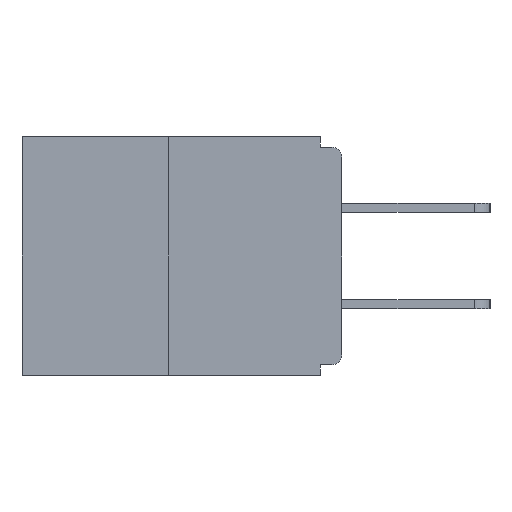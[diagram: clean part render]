
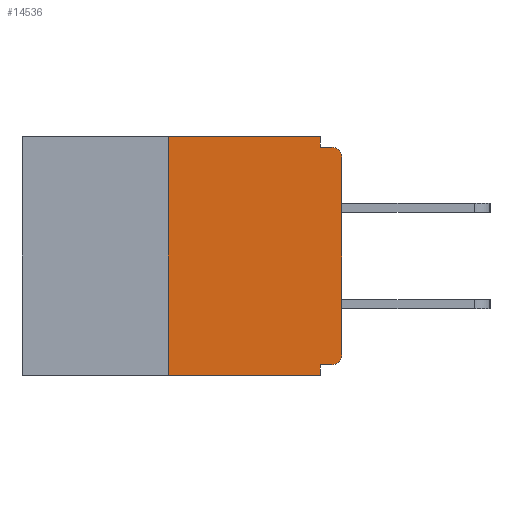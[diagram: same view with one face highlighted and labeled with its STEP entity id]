
A CAD part, left-side view. The second image highlights one B-rep face of the part: STEP entity #14536.
In plain terms, the highlighted planar face has unit normal (-1, 0, 0).
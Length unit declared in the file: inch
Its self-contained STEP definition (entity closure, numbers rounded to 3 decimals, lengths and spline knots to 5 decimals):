
#275 = CARTESIAN_POINT ( 'NONE',  ( 0., 0.031, -0.343 ) ) ;
#587 = VECTOR ( 'NONE', #9643, 39.37008 ) ;
#678 = CARTESIAN_POINT ( 'NONE',  ( 0., 0.031, 0. ) ) ;
#707 = VERTEX_POINT ( 'NONE', #5358 ) ;
#1022 = PLANE ( 'NONE',  #9629 ) ;
#1373 = LINE ( 'NONE', #3670, #10844 ) ;
#1382 = EDGE_CURVE ( 'NONE', #10018, #707, #10450, .T. ) ;
#1393 = VERTEX_POINT ( 'NONE', #15628 ) ;
#1470 = LINE ( 'NONE', #678, #11125 ) ;
#1622 = EDGE_CURVE ( 'NONE', #1393, #10018, #7675, .T. ) ;
#1637 = EDGE_CURVE ( 'NONE', #4875, #10970, #4033, .T. ) ;
#1712 = EDGE_CURVE ( 'NONE', #7750, #13400, #11394, .T. ) ;
#1716 = DIRECTION ( 'NONE',  ( 0., -1., 0. ) ) ;
#2044 = CARTESIAN_POINT ( 'NONE',  ( 0., 0.46, 0. ) ) ;
#2189 = DIRECTION ( 'NONE',  ( 1., 0., 0. ) ) ;
#2559 = VECTOR ( 'NONE', #3470, 39.37008 ) ;
#2669 = CARTESIAN_POINT ( 'NONE',  ( 0., 0.031, -0.343 ) ) ;
#2687 = VERTEX_POINT ( 'NONE', #275 ) ;
#2695 = VECTOR ( 'NONE', #5505, 39.37008 ) ;
#3091 = EDGE_CURVE ( 'NONE', #4007, #2687, #11808, .T. ) ;
#3470 = DIRECTION ( 'NONE',  ( 0., 0., -1. ) ) ;
#3670 = CARTESIAN_POINT ( 'NONE',  ( 0., 0., -0.328 ) ) ;
#3882 = FACE_OUTER_BOUND ( 'NONE', #10407, .T. ) ;
#4007 = VERTEX_POINT ( 'NONE', #11695 ) ;
#4033 = LINE ( 'NONE', #10534, #9449 ) ;
#4038 = DIRECTION ( 'NONE',  ( 0., 0., -1. ) ) ;
#4139 = CARTESIAN_POINT ( 'NONE',  ( 0., 0.015, -0.03 ) ) ;
#4372 = VERTEX_POINT ( 'NONE', #10000 ) ;
#4607 = LINE ( 'NONE', #12902, #6707 ) ;
#4738 = ORIENTED_EDGE ( 'NONE', *, *, #8450, .F. ) ;
#4875 = VERTEX_POINT ( 'NONE', #13530 ) ;
#5358 = CARTESIAN_POINT ( 'NONE',  ( 0., 0., -0.03 ) ) ;
#5442 = ORIENTED_EDGE ( 'NONE', *, *, #15208, .F. ) ;
#5505 = DIRECTION ( 'NONE',  ( 0., 0., 1. ) ) ;
#5766 = CARTESIAN_POINT ( 'NONE',  ( 0., 0.25, -0.343 ) ) ;
#5880 = CARTESIAN_POINT ( 'NONE',  ( 0., 0.46, 0. ) ) ;
#6170 = ORIENTED_EDGE ( 'NONE', *, *, #11322, .F. ) ;
#6456 = CARTESIAN_POINT ( 'NONE',  ( 0., 0.015, -0.313 ) ) ;
#6502 = ORIENTED_EDGE ( 'NONE', *, *, #3091, .F. ) ;
#6707 = VECTOR ( 'NONE', #1716, 39.37008 ) ;
#7675 = CIRCLE ( 'NONE', #8527, 0.015 ) ;
#7750 = VERTEX_POINT ( 'NONE', #5766 ) ;
#8117 = DIRECTION ( 'NONE',  ( 0., -1., 0. ) ) ;
#8254 = AXIS2_PLACEMENT_3D ( 'NONE', #4139, #11453, #4038 ) ;
#8450 = EDGE_CURVE ( 'NONE', #4372, #4875, #1470, .T. ) ;
#8527 = AXIS2_PLACEMENT_3D ( 'NONE', #6456, #13016, #15363 ) ;
#9134 = ORIENTED_EDGE ( 'NONE', *, *, #11204, .T. ) ;
#9315 = CARTESIAN_POINT ( 'NONE',  ( 0., 0., -0.313 ) ) ;
#9449 = VECTOR ( 'NONE', #11766, 39.37008 ) ;
#9629 = AXIS2_PLACEMENT_3D ( 'NONE', #5880, #2189, #12071 ) ;
#9643 = DIRECTION ( 'NONE',  ( 0., 0., 1. ) ) ;
#10000 = CARTESIAN_POINT ( 'NONE',  ( 0., 0.031, 0. ) ) ;
#10018 = VERTEX_POINT ( 'NONE', #9315 ) ;
#10353 = ORIENTED_EDGE ( 'NONE', *, *, #1622, .T. ) ;
#10407 = EDGE_LOOP ( 'NONE', ( #6170, #15580, #14016, #6502, #5442, #10353, #13930, #9134, #15833, #4738 ) ) ;
#10450 = LINE ( 'NONE', #15672, #587 ) ;
#10534 = CARTESIAN_POINT ( 'NONE',  ( 0., 0., -0.015 ) ) ;
#10844 = VECTOR ( 'NONE', #13733, 39.37008 ) ;
#10970 = VERTEX_POINT ( 'NONE', #12107 ) ;
#11125 = VECTOR ( 'NONE', #11835, 39.37008 ) ;
#11204 = EDGE_CURVE ( 'NONE', #707, #10970, #15153, .T. ) ;
#11322 = EDGE_CURVE ( 'NONE', #13400, #4372, #13216, .T. ) ;
#11394 = LINE ( 'NONE', #14227, #2695 ) ;
#11453 = DIRECTION ( 'NONE',  ( -1., 0., 0. ) ) ;
#11651 = CARTESIAN_POINT ( 'NONE',  ( 0., 0.25, 0. ) ) ;
#11695 = CARTESIAN_POINT ( 'NONE',  ( 0., 0.031, -0.328 ) ) ;
#11766 = DIRECTION ( 'NONE',  ( 0., -1., 0. ) ) ;
#11808 = LINE ( 'NONE', #2669, #2559 ) ;
#11835 = DIRECTION ( 'NONE',  ( 0., 0., -1. ) ) ;
#12071 = DIRECTION ( 'NONE',  ( 0., 0., -1. ) ) ;
#12073 = VECTOR ( 'NONE', #8117, 39.37008 ) ;
#12107 = CARTESIAN_POINT ( 'NONE',  ( 0., 0.015, -0.015 ) ) ;
#12902 = CARTESIAN_POINT ( 'NONE',  ( 0., 0.46, -0.343 ) ) ;
#13016 = DIRECTION ( 'NONE',  ( -1., 0., 0. ) ) ;
#13216 = LINE ( 'NONE', #2044, #12073 ) ;
#13400 = VERTEX_POINT ( 'NONE', #11651 ) ;
#13530 = CARTESIAN_POINT ( 'NONE',  ( 0., 0.031, -0.015 ) ) ;
#13733 = DIRECTION ( 'NONE',  ( 0., 1., 0. ) ) ;
#13930 = ORIENTED_EDGE ( 'NONE', *, *, #1382, .T. ) ;
#14016 = ORIENTED_EDGE ( 'NONE', *, *, #14947, .T. ) ;
#14227 = CARTESIAN_POINT ( 'NONE',  ( 0., 0.25, 0. ) ) ;
#14536 = ADVANCED_FACE ( 'NONE', ( #3882 ), #1022, .F. ) ;
#14947 = EDGE_CURVE ( 'NONE', #7750, #2687, #4607, .T. ) ;
#15153 = CIRCLE ( 'NONE', #8254, 0.015 ) ;
#15208 = EDGE_CURVE ( 'NONE', #1393, #4007, #1373, .T. ) ;
#15363 = DIRECTION ( 'NONE',  ( 0., 0., -1. ) ) ;
#15580 = ORIENTED_EDGE ( 'NONE', *, *, #1712, .F. ) ;
#15628 = CARTESIAN_POINT ( 'NONE',  ( 0., 0.015, -0.328 ) ) ;
#15672 = CARTESIAN_POINT ( 'NONE',  ( 0., 0., 0. ) ) ;
#15833 = ORIENTED_EDGE ( 'NONE', *, *, #1637, .F. ) ;
